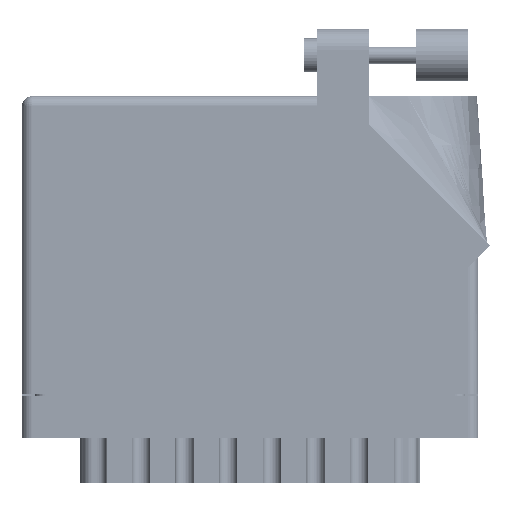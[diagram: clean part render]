
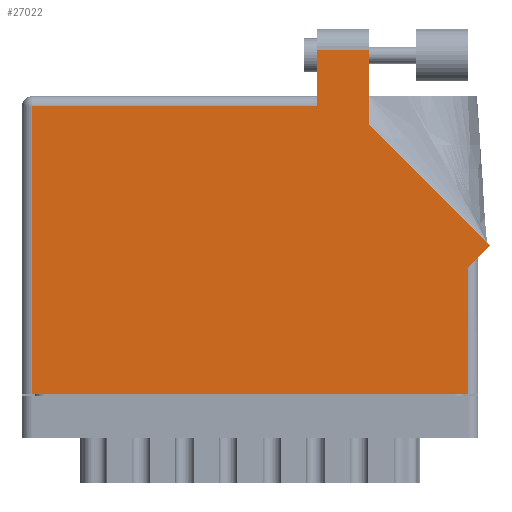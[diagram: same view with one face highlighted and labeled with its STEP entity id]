
A CAD part, front view. The second image highlights one B-rep face of the part: STEP entity #27022.
In plain terms, the highlighted face is planar.
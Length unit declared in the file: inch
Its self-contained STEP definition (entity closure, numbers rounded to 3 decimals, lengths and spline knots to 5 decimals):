
#196 = VERTEX_POINT ( 'NONE', #12915 ) ;
#398 = EDGE_CURVE ( 'NONE', #16760, #5469, #64098, .T. ) ;
#501 = EDGE_CURVE ( 'NONE', #11584, #44170, #72918, .T. ) ;
#1113 = VECTOR ( 'NONE', #6486, 39.37008 ) ;
#1880 = CARTESIAN_POINT ( 'NONE',  ( 0., 0., 0. ) ) ;
#2613 = VERTEX_POINT ( 'NONE', #31785 ) ;
#2996 = LINE ( 'NONE', #35851, #55816 ) ;
#4303 = EDGE_LOOP ( 'NONE', ( #34729, #8763, #36196, #64342, #32506, #59300, #12702, #50869, #50251 ) ) ;
#5469 = VERTEX_POINT ( 'NONE', #20491 ) ;
#5839 = CARTESIAN_POINT ( 'NONE',  ( 0.062, 1.713, 0. ) ) ;
#6486 = DIRECTION ( 'NONE',  ( 0., -1., 0. ) ) ;
#7915 = DIRECTION ( 'NONE',  ( -1., 0., 0. ) ) ;
#8763 = ORIENTED_EDGE ( 'NONE', *, *, #25984, .T. ) ;
#10412 = CARTESIAN_POINT ( 'NONE',  ( 2.78871, 0.88571, 0. ) ) ;
#11584 = VERTEX_POINT ( 'NONE', #10412 ) ;
#11902 = EDGE_CURVE ( 'NONE', #44170, #52682, #53032, .T. ) ;
#12702 = ORIENTED_EDGE ( 'NONE', *, *, #26749, .T. ) ;
#12915 = CARTESIAN_POINT ( 'NONE',  ( 2.656, 0.753, 0. ) ) ;
#14022 = DIRECTION ( 'NONE',  ( 0., -1., 0. ) ) ;
#16760 = VERTEX_POINT ( 'NONE', #66804 ) ;
#18598 = CARTESIAN_POINT ( 'NONE',  ( 2.718, 0.815, 0. ) ) ;
#19377 = LINE ( 'NONE', #41710, #31765 ) ;
#20491 = CARTESIAN_POINT ( 'NONE',  ( 2.656, 0., 0. ) ) ;
#20523 = DIRECTION ( 'NONE',  ( 0., 0., -1. ) ) ;
#21405 = FACE_OUTER_BOUND ( 'NONE', #4303, .T. ) ;
#23329 = AXIS2_PLACEMENT_3D ( 'NONE', #32134, #20523, #66272 ) ;
#23845 = VERTEX_POINT ( 'NONE', #32636 ) ;
#24955 = LINE ( 'NONE', #39797, #1113 ) ;
#25408 = DIRECTION ( 'NONE',  ( 0., 1., 0. ) ) ;
#25984 = EDGE_CURVE ( 'NONE', #52682, #23845, #19377, .T. ) ;
#26688 = PLANE ( 'NONE',  #23329 ) ;
#26749 = EDGE_CURVE ( 'NONE', #5469, #196, #2996, .T. ) ;
#27022 = ADVANCED_FACE ( 'NONE', ( #21405 ), #26688, .F. ) ;
#29956 = DIRECTION ( 'NONE',  ( 0.707, 0.707, 0. ) ) ;
#30498 = DIRECTION ( 'NONE',  ( 1., 0., 0. ) ) ;
#31195 = EDGE_CURVE ( 'NONE', #196, #11584, #44706, .T. ) ;
#31765 = VECTOR ( 'NONE', #7915, 39.37008 ) ;
#31785 = CARTESIAN_POINT ( 'NONE',  ( 1.758, 1.713, 0. ) ) ;
#32134 = CARTESIAN_POINT ( 'NONE',  ( 0., 1.775, 0. ) ) ;
#32506 = ORIENTED_EDGE ( 'NONE', *, *, #35048, .T. ) ;
#32636 = CARTESIAN_POINT ( 'NONE',  ( 1.758, 2.05, 0. ) ) ;
#34729 = ORIENTED_EDGE ( 'NONE', *, *, #11902, .T. ) ;
#35048 = EDGE_CURVE ( 'NONE', #70423, #16760, #24955, .T. ) ;
#35851 = CARTESIAN_POINT ( 'NONE',  ( 2.656, 0.815, 0. ) ) ;
#36196 = ORIENTED_EDGE ( 'NONE', *, *, #48937, .T. ) ;
#37620 = CARTESIAN_POINT ( 'NONE',  ( 0., 1.713, 0. ) ) ;
#38579 = VECTOR ( 'NONE', #29956, 39.37008 ) ;
#39797 = CARTESIAN_POINT ( 'NONE',  ( 0.062, 0., 0. ) ) ;
#41692 = CARTESIAN_POINT ( 'NONE',  ( 1.758, 1.775, 0. ) ) ;
#41710 = CARTESIAN_POINT ( 'NONE',  ( 1.758, 2.05, 0. ) ) ;
#42764 = CARTESIAN_POINT ( 'NONE',  ( 2.78871, 0.88571, 0. ) ) ;
#43034 = VECTOR ( 'NONE', #54316, 39.37008 ) ;
#43279 = DIRECTION ( 'NONE',  ( -1., 0., 0. ) ) ;
#44170 = VERTEX_POINT ( 'NONE', #60150 ) ;
#44706 = LINE ( 'NONE', #18598, #38579 ) ;
#45258 = CARTESIAN_POINT ( 'NONE',  ( 2.065, 2.05, 0. ) ) ;
#45303 = EDGE_CURVE ( 'NONE', #2613, #70423, #58721, .T. ) ;
#48937 = EDGE_CURVE ( 'NONE', #23845, #2613, #71794, .T. ) ;
#49061 = VECTOR ( 'NONE', #43279, 39.37008 ) ;
#50077 = VECTOR ( 'NONE', #30498, 39.37008 ) ;
#50251 = ORIENTED_EDGE ( 'NONE', *, *, #501, .T. ) ;
#50869 = ORIENTED_EDGE ( 'NONE', *, *, #31195, .T. ) ;
#51266 = VECTOR ( 'NONE', #25408, 39.37008 ) ;
#52682 = VERTEX_POINT ( 'NONE', #45258 ) ;
#53009 = CARTESIAN_POINT ( 'NONE',  ( 2.065, 1.60942, 0. ) ) ;
#53032 = LINE ( 'NONE', #53009, #51266 ) ;
#54316 = DIRECTION ( 'NONE',  ( -0.707, 0.707, 0. ) ) ;
#55816 = VECTOR ( 'NONE', #57738, 39.37008 ) ;
#57738 = DIRECTION ( 'NONE',  ( 0., 1., 0. ) ) ;
#58721 = LINE ( 'NONE', #37620, #49061 ) ;
#59300 = ORIENTED_EDGE ( 'NONE', *, *, #398, .T. ) ;
#60150 = CARTESIAN_POINT ( 'NONE',  ( 2.065, 1.60942, 0. ) ) ;
#64098 = LINE ( 'NONE', #1880, #50077 ) ;
#64342 = ORIENTED_EDGE ( 'NONE', *, *, #45303, .T. ) ;
#66272 = DIRECTION ( 'NONE',  ( -1., 0., 0. ) ) ;
#66493 = VECTOR ( 'NONE', #14022, 39.37008 ) ;
#66804 = CARTESIAN_POINT ( 'NONE',  ( 0.062, 0., 0. ) ) ;
#70423 = VERTEX_POINT ( 'NONE', #5839 ) ;
#71794 = LINE ( 'NONE', #41692, #66493 ) ;
#72918 = LINE ( 'NONE', #42764, #43034 ) ;
